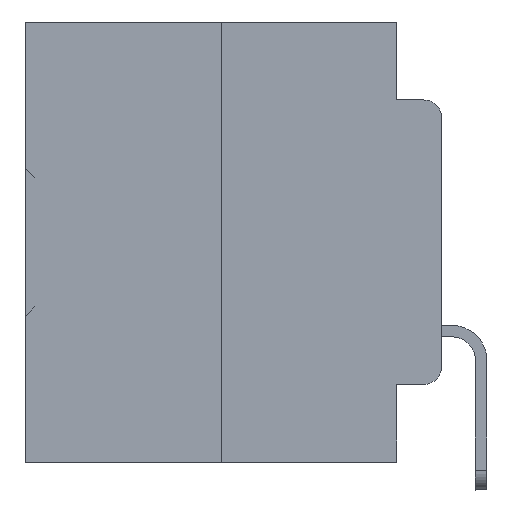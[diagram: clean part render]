
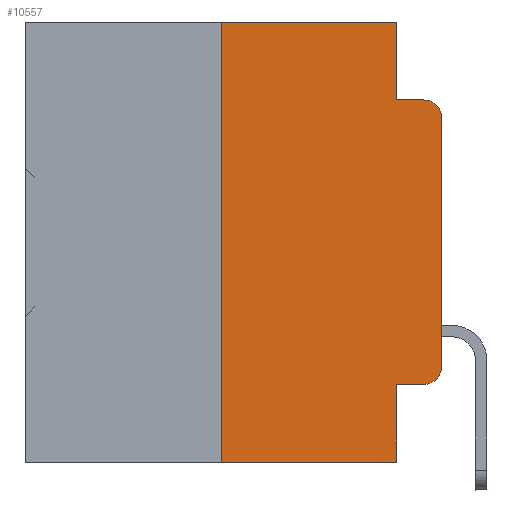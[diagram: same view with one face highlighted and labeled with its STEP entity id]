
A CAD part, left-side view. The second image highlights one B-rep face of the part: STEP entity #10557.
In plain terms, the highlighted planar face has unit normal (-1, 0, 0).
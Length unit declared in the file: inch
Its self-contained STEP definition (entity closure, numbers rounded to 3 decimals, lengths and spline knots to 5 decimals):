
#186 = EDGE_CURVE ( 'NONE', #35803, #19389, #5233, .T. ) ;
#383 = CARTESIAN_POINT ( 'NONE',  ( 0., 0.051, 0. ) ) ;
#863 = DIRECTION ( 'NONE',  ( 0., -1., 0. ) ) ;
#1550 = ORIENTED_EDGE ( 'NONE', *, *, #12682, .F. ) ;
#2200 = LINE ( 'NONE', #34752, #20977 ) ;
#2726 = DIRECTION ( 'NONE',  ( 0., -1., 0. ) ) ;
#2768 = LINE ( 'NONE', #18439, #21227 ) ;
#2916 = DIRECTION ( 'NONE',  ( -1., 0., 0. ) ) ;
#3299 = CARTESIAN_POINT ( 'NONE',  ( 0., 0.02, -0.1085 ) ) ;
#3640 = VECTOR ( 'NONE', #33705, 39.37008 ) ;
#4104 = EDGE_CURVE ( 'NONE', #7272, #22648, #23859, .T. ) ;
#4401 = CIRCLE ( 'NONE', #20064, 0.02 ) ;
#4999 = DIRECTION ( 'NONE',  ( 0., 0., 1. ) ) ;
#5233 = LINE ( 'NONE', #23051, #9310 ) ;
#5517 = VECTOR ( 'NONE', #2726, 39.37008 ) ;
#5628 = EDGE_CURVE ( 'NONE', #7272, #22518, #22468, .T. ) ;
#6326 = ORIENTED_EDGE ( 'NONE', *, *, #5628, .F. ) ;
#6492 = CIRCLE ( 'NONE', #28393, 0.02 ) ;
#7272 = VERTEX_POINT ( 'NONE', #15866 ) ;
#7525 = VERTEX_POINT ( 'NONE', #14840 ) ;
#8067 = VERTEX_POINT ( 'NONE', #18677 ) ;
#8176 = CARTESIAN_POINT ( 'NONE',  ( 0., 0.25, 0. ) ) ;
#8567 = CARTESIAN_POINT ( 'NONE',  ( 0., 0.051, -0.5 ) ) ;
#8712 = ORIENTED_EDGE ( 'NONE', *, *, #18947, .T. ) ;
#9273 = DIRECTION ( 'NONE',  ( 0., 0., -1. ) ) ;
#9310 = VECTOR ( 'NONE', #37597, 39.37008 ) ;
#9374 = ORIENTED_EDGE ( 'NONE', *, *, #16112, .F. ) ;
#9953 = CARTESIAN_POINT ( 'NONE',  ( 0., 0.25, 0. ) ) ;
#10557 = ADVANCED_FACE ( 'NONE', ( #32238 ), #22979, .F. ) ;
#12682 = EDGE_CURVE ( 'NONE', #12805, #20090, #2200, .T. ) ;
#12805 = VERTEX_POINT ( 'NONE', #27068 ) ;
#13786 = CARTESIAN_POINT ( 'NONE',  ( 0., 0.473, 0. ) ) ;
#14840 = CARTESIAN_POINT ( 'NONE',  ( 0., 0., -0.1085 ) ) ;
#15461 = CARTESIAN_POINT ( 'NONE',  ( 0., 0.02, -0.4115 ) ) ;
#15866 = CARTESIAN_POINT ( 'NONE',  ( 0., 0.25, -0.5 ) ) ;
#16112 = EDGE_CURVE ( 'NONE', #22518, #18511, #33619, .T. ) ;
#16559 = VECTOR ( 'NONE', #34466, 39.37008 ) ;
#17544 = ORIENTED_EDGE ( 'NONE', *, *, #23312, .T. ) ;
#17861 = DIRECTION ( 'NONE',  ( 0., 0., -1. ) ) ;
#18118 = VECTOR ( 'NONE', #863, 39.37008 ) ;
#18439 = CARTESIAN_POINT ( 'NONE',  ( 0., 0.051, 0. ) ) ;
#18511 = VERTEX_POINT ( 'NONE', #20541 ) ;
#18677 = CARTESIAN_POINT ( 'NONE',  ( 0., 0., -0.3915 ) ) ;
#18947 = EDGE_CURVE ( 'NONE', #19389, #8067, #4401, .T. ) ;
#19389 = VERTEX_POINT ( 'NONE', #15461 ) ;
#19445 = DIRECTION ( 'NONE',  ( 0., -1., 0. ) ) ;
#20064 = AXIS2_PLACEMENT_3D ( 'NONE', #21604, #30279, #9273 ) ;
#20090 = VERTEX_POINT ( 'NONE', #32473 ) ;
#20098 = LINE ( 'NONE', #22806, #36150 ) ;
#20187 = ORIENTED_EDGE ( 'NONE', *, *, #4104, .T. ) ;
#20541 = CARTESIAN_POINT ( 'NONE',  ( 0., 0.051, 0. ) ) ;
#20977 = VECTOR ( 'NONE', #19445, 39.37008 ) ;
#21227 = VECTOR ( 'NONE', #17861, 39.37008 ) ;
#21604 = CARTESIAN_POINT ( 'NONE',  ( 0., 0.02, -0.3915 ) ) ;
#21771 = ORIENTED_EDGE ( 'NONE', *, *, #186, .T. ) ;
#22468 = LINE ( 'NONE', #8176, #16559 ) ;
#22518 = VERTEX_POINT ( 'NONE', #9953 ) ;
#22648 = VERTEX_POINT ( 'NONE', #8567 ) ;
#22806 = CARTESIAN_POINT ( 'NONE',  ( 0., 0., 0. ) ) ;
#22813 = AXIS2_PLACEMENT_3D ( 'NONE', #13786, #37320, #37723 ) ;
#22979 = PLANE ( 'NONE',  #22813 ) ;
#23051 = CARTESIAN_POINT ( 'NONE',  ( 0., 0.051, -0.4115 ) ) ;
#23312 = EDGE_CURVE ( 'NONE', #8067, #7525, #20098, .T. ) ;
#23859 = LINE ( 'NONE', #26830, #5517 ) ;
#24352 = EDGE_LOOP ( 'NONE', ( #17544, #37640, #1550, #38408, #9374, #6326, #20187, #26511, #21771, #8712 ) ) ;
#24379 = EDGE_CURVE ( 'NONE', #18511, #12805, #36632, .T. ) ;
#25146 = CARTESIAN_POINT ( 'NONE',  ( 0., 0.473, 0. ) ) ;
#26511 = ORIENTED_EDGE ( 'NONE', *, *, #38585, .F. ) ;
#26830 = CARTESIAN_POINT ( 'NONE',  ( 0., 0.473, -0.5 ) ) ;
#27068 = CARTESIAN_POINT ( 'NONE',  ( 0., 0.051, -0.0885 ) ) ;
#28393 = AXIS2_PLACEMENT_3D ( 'NONE', #3299, #2916, #35670 ) ;
#30279 = DIRECTION ( 'NONE',  ( -1., 0., 0. ) ) ;
#31005 = CARTESIAN_POINT ( 'NONE',  ( 0., 0.051, -0.4115 ) ) ;
#31122 = EDGE_CURVE ( 'NONE', #7525, #20090, #6492, .T. ) ;
#32238 = FACE_OUTER_BOUND ( 'NONE', #24352, .T. ) ;
#32473 = CARTESIAN_POINT ( 'NONE',  ( 0., 0.02, -0.0885 ) ) ;
#33619 = LINE ( 'NONE', #25146, #18118 ) ;
#33705 = DIRECTION ( 'NONE',  ( 0., 0., -1. ) ) ;
#34466 = DIRECTION ( 'NONE',  ( 0., 0., 1. ) ) ;
#34752 = CARTESIAN_POINT ( 'NONE',  ( 0., 0.051, -0.0885 ) ) ;
#35670 = DIRECTION ( 'NONE',  ( 0., 0., -1. ) ) ;
#35803 = VERTEX_POINT ( 'NONE', #31005 ) ;
#36150 = VECTOR ( 'NONE', #4999, 39.37008 ) ;
#36632 = LINE ( 'NONE', #383, #3640 ) ;
#37320 = DIRECTION ( 'NONE',  ( 1., 0., 0. ) ) ;
#37597 = DIRECTION ( 'NONE',  ( 0., -1., 0. ) ) ;
#37640 = ORIENTED_EDGE ( 'NONE', *, *, #31122, .T. ) ;
#37723 = DIRECTION ( 'NONE',  ( 0., 0., -1. ) ) ;
#38408 = ORIENTED_EDGE ( 'NONE', *, *, #24379, .F. ) ;
#38585 = EDGE_CURVE ( 'NONE', #35803, #22648, #2768, .T. ) ;
